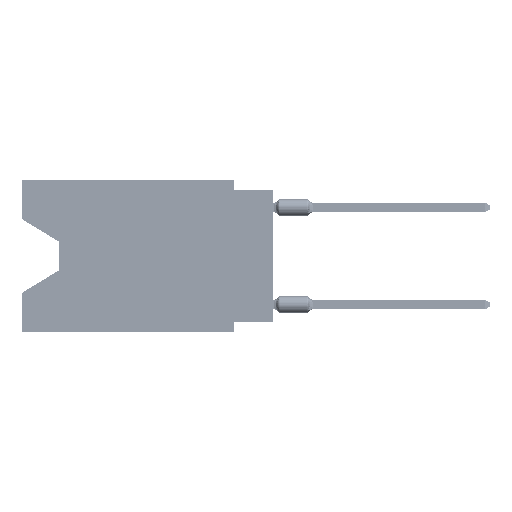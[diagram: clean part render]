
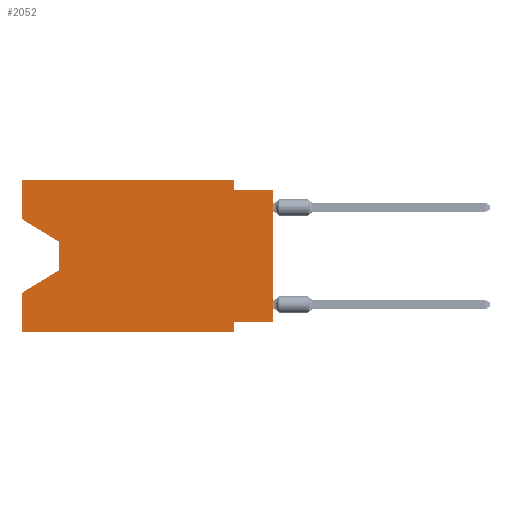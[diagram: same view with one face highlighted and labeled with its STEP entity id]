
A CAD part, left-side view. The second image highlights one B-rep face of the part: STEP entity #2052.
In plain terms, the highlighted planar face has unit normal (-1, 0, 0).
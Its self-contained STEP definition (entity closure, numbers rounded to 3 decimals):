
#482 = VERTEX_POINT ( 'NONE', #19607 ) ;
#787 = EDGE_CURVE ( 'NONE', #4106, #16998, #35710, .T. ) ;
#2017 = VECTOR ( 'NONE', #47077, 1000. ) ;
#2052 = ADVANCED_FACE ( 'NONE', ( #24923 ), #61100, .F. ) ;
#3257 = LINE ( 'NONE', #32112, #69363 ) ;
#4106 = VERTEX_POINT ( 'NONE', #6690 ) ;
#4490 = ORIENTED_EDGE ( 'NONE', *, *, #787, .F. ) ;
#4874 = VECTOR ( 'NONE', #8622, 1000. ) ;
#5904 = CARTESIAN_POINT ( 'NONE',  ( 0., 16.383, 0. ) ) ;
#6690 = CARTESIAN_POINT ( 'NONE',  ( 0., 0., -9.271 ) ) ;
#7621 = VERTEX_POINT ( 'NONE', #27217 ) ;
#8021 = EDGE_CURVE ( 'NONE', #7621, #26440, #69727, .T. ) ;
#8622 = DIRECTION ( 'NONE',  ( 0., 0., -1. ) ) ;
#9774 = CARTESIAN_POINT ( 'NONE',  ( 0., 16.383, -9.906 ) ) ;
#9799 = DIRECTION ( 'NONE',  ( 0., 0., -1. ) ) ;
#10043 = DIRECTION ( 'NONE',  ( 0., 0., 1. ) ) ;
#10195 = ORIENTED_EDGE ( 'NONE', *, *, #37416, .T. ) ;
#10431 = EDGE_CURVE ( 'NONE', #59051, #27346, #23796, .T. ) ;
#12044 = CARTESIAN_POINT ( 'NONE',  ( 0., 13.97, -5.893 ) ) ;
#12904 = CARTESIAN_POINT ( 'NONE',  ( 0., 2.54, -0.635 ) ) ;
#12996 = DIRECTION ( 'NONE',  ( 1., 0., 0. ) ) ;
#13067 = VECTOR ( 'NONE', #27933, 1000. ) ;
#15909 = EDGE_CURVE ( 'NONE', #27346, #66301, #3257, .T. ) ;
#16983 = ORIENTED_EDGE ( 'NONE', *, *, #29384, .T. ) ;
#16998 = VERTEX_POINT ( 'NONE', #64689 ) ;
#18738 = CARTESIAN_POINT ( 'NONE',  ( 0., 16.383, -2.546 ) ) ;
#19607 = CARTESIAN_POINT ( 'NONE',  ( 0., 16.383, -9.906 ) ) ;
#20198 = ORIENTED_EDGE ( 'NONE', *, *, #10431, .F. ) ;
#20650 = CARTESIAN_POINT ( 'NONE',  ( 0., 16.383, -7.36 ) ) ;
#21552 = EDGE_CURVE ( 'NONE', #47612, #59096, #56622, .T. ) ;
#21600 = AXIS2_PLACEMENT_3D ( 'NONE', #60339, #12996, #54188 ) ;
#22460 = VERTEX_POINT ( 'NONE', #20650 ) ;
#22822 = EDGE_CURVE ( 'NONE', #16998, #65028, #32867, .T. ) ;
#22905 = LINE ( 'NONE', #46001, #13067 ) ;
#23763 = VECTOR ( 'NONE', #29928, 1000. ) ;
#23796 = LINE ( 'NONE', #53437, #33333 ) ;
#24030 = EDGE_CURVE ( 'NONE', #482, #65028, #55586, .T. ) ;
#24039 = CARTESIAN_POINT ( 'NONE',  ( 0., 16.383, -2.546 ) ) ;
#24554 = LINE ( 'NONE', #48040, #69708 ) ;
#24923 = FACE_OUTER_BOUND ( 'NONE', #48359, .T. ) ;
#25217 = ORIENTED_EDGE ( 'NONE', *, *, #65344, .F. ) ;
#25337 = ORIENTED_EDGE ( 'NONE', *, *, #22822, .F. ) ;
#26440 = VERTEX_POINT ( 'NONE', #12044 ) ;
#26917 = VECTOR ( 'NONE', #9799, 1000. ) ;
#27217 = CARTESIAN_POINT ( 'NONE',  ( 0., 13.97, -4.013 ) ) ;
#27235 = ORIENTED_EDGE ( 'NONE', *, *, #8021, .T. ) ;
#27346 = VERTEX_POINT ( 'NONE', #12904 ) ;
#27933 = DIRECTION ( 'NONE',  ( 0., 0., 1. ) ) ;
#28903 = VECTOR ( 'NONE', #37479, 1000. ) ;
#29384 = EDGE_CURVE ( 'NONE', #26440, #22460, #46644, .T. ) ;
#29928 = DIRECTION ( 'NONE',  ( 0., 1., 0. ) ) ;
#32112 = CARTESIAN_POINT ( 'NONE',  ( 0., 0., -0.635 ) ) ;
#32867 = LINE ( 'NONE', #33235, #4874 ) ;
#33032 = VECTOR ( 'NONE', #58560, 1000. ) ;
#33235 = CARTESIAN_POINT ( 'NONE',  ( 0., 2.54, -9.906 ) ) ;
#33333 = VECTOR ( 'NONE', #36485, 1000. ) ;
#34281 = CARTESIAN_POINT ( 'NONE',  ( 0., 16.383, 0. ) ) ;
#35143 = LINE ( 'NONE', #5904, #2017 ) ;
#35710 = LINE ( 'NONE', #59182, #23763 ) ;
#36485 = DIRECTION ( 'NONE',  ( 0., 0., -1. ) ) ;
#37416 = EDGE_CURVE ( 'NONE', #47612, #7621, #59827, .T. ) ;
#37479 = DIRECTION ( 'NONE',  ( 0., -0.855, -0.519 ) ) ;
#44082 = ORIENTED_EDGE ( 'NONE', *, *, #15909, .F. ) ;
#46001 = CARTESIAN_POINT ( 'NONE',  ( 0., 16.383, 0. ) ) ;
#46644 = LINE ( 'NONE', #71618, #33032 ) ;
#47077 = DIRECTION ( 'NONE',  ( 0., -1., 0. ) ) ;
#47612 = VERTEX_POINT ( 'NONE', #18738 ) ;
#48040 = CARTESIAN_POINT ( 'NONE',  ( 0., 0., 0. ) ) ;
#48359 = EDGE_LOOP ( 'NONE', ( #10195, #27235, #16983, #25217, #53674, #25337, #4490, #65194, #44082, #20198, #69744, #58346 ) ) ;
#49832 = DIRECTION ( 'NONE',  ( 0., -1., 0. ) ) ;
#50451 = VECTOR ( 'NONE', #10043, 1000. ) ;
#53004 = CARTESIAN_POINT ( 'NONE',  ( 0., 2.54, -9.906 ) ) ;
#53437 = CARTESIAN_POINT ( 'NONE',  ( 0., 2.54, 0. ) ) ;
#53674 = ORIENTED_EDGE ( 'NONE', *, *, #24030, .T. ) ;
#54188 = DIRECTION ( 'NONE',  ( 0., 0., -1. ) ) ;
#55586 = LINE ( 'NONE', #9774, #66467 ) ;
#56622 = LINE ( 'NONE', #34281, #50451 ) ;
#56725 = DIRECTION ( 'NONE',  ( 0., -1., 0. ) ) ;
#58346 = ORIENTED_EDGE ( 'NONE', *, *, #21552, .F. ) ;
#58560 = DIRECTION ( 'NONE',  ( 0., 0.855, -0.519 ) ) ;
#59051 = VERTEX_POINT ( 'NONE', #73490 ) ;
#59096 = VERTEX_POINT ( 'NONE', #75385 ) ;
#59182 = CARTESIAN_POINT ( 'NONE',  ( 0., 0., -9.271 ) ) ;
#59827 = LINE ( 'NONE', #24039, #28903 ) ;
#60339 = CARTESIAN_POINT ( 'NONE',  ( 0., 16.383, 0. ) ) ;
#61100 = PLANE ( 'NONE',  #21600 ) ;
#64689 = CARTESIAN_POINT ( 'NONE',  ( 0., 2.54, -9.271 ) ) ;
#65028 = VERTEX_POINT ( 'NONE', #53004 ) ;
#65194 = ORIENTED_EDGE ( 'NONE', *, *, #66680, .T. ) ;
#65344 = EDGE_CURVE ( 'NONE', #482, #22460, #22905, .T. ) ;
#65714 = EDGE_CURVE ( 'NONE', #59096, #59051, #35143, .T. ) ;
#66301 = VERTEX_POINT ( 'NONE', #68862 ) ;
#66467 = VECTOR ( 'NONE', #56725, 1000. ) ;
#66680 = EDGE_CURVE ( 'NONE', #4106, #66301, #24554, .T. ) ;
#68862 = CARTESIAN_POINT ( 'NONE',  ( 0., 0., -0.635 ) ) ;
#69363 = VECTOR ( 'NONE', #49832, 1000. ) ;
#69708 = VECTOR ( 'NONE', #71500, 1000. ) ;
#69727 = LINE ( 'NONE', #74049, #26917 ) ;
#69744 = ORIENTED_EDGE ( 'NONE', *, *, #65714, .F. ) ;
#71500 = DIRECTION ( 'NONE',  ( 0., 0., 1. ) ) ;
#71618 = CARTESIAN_POINT ( 'NONE',  ( 0., 13.97, -5.893 ) ) ;
#73490 = CARTESIAN_POINT ( 'NONE',  ( 0., 2.54, 0. ) ) ;
#74049 = CARTESIAN_POINT ( 'NONE',  ( 0., 13.97, -4.013 ) ) ;
#75385 = CARTESIAN_POINT ( 'NONE',  ( 0., 16.383, 0. ) ) ;
